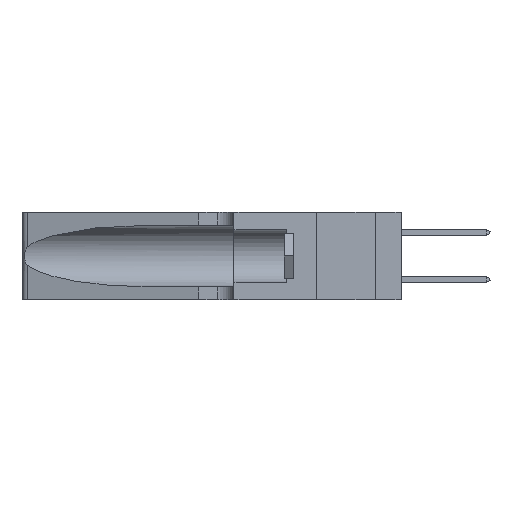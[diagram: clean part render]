
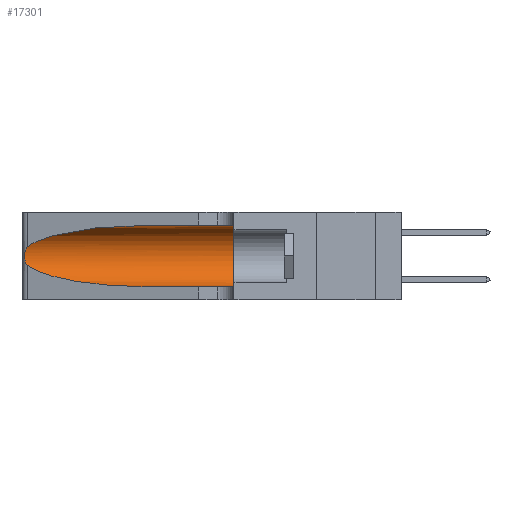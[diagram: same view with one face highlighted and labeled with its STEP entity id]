
A CAD part, left-side view. The second image highlights one B-rep face of the part: STEP entity #17301.
In plain terms, the highlighted cylindrical face has radius 3.308 mm (diameter 6.617 mm), a partial arc.
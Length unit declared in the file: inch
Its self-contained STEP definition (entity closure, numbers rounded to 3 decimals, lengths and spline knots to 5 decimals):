
#1300 = LINE ( 'NONE', #16439, #38220 ) ;
#2015 = VERTEX_POINT ( 'NONE', #31991 ) ;
#2407 = DIRECTION ( 'NONE',  ( 0., -1., 0. ) ) ;
#2857 = CARTESIAN_POINT ( 'NONE',  ( 0.26017, 1.23833, 0.17102 ) ) ;
#2988 = VECTOR ( 'NONE', #34786, 39.37008 ) ;
#3005 = CARTESIAN_POINT ( 'NONE',  ( 0.25555, 1.22994, 0.2215 ) ) ;
#3020 = ORIENTED_EDGE ( 'NONE', *, *, #15804, .T. ) ;
#4211 = ORIENTED_EDGE ( 'NONE', *, *, #12583, .T. ) ;
#4261 = VERTEX_POINT ( 'NONE', #44285 ) ;
#5601 = CARTESIAN_POINT ( 'NONE',  ( 0.1305, 1.61858, 0.185 ) ) ;
#5669 = ORIENTED_EDGE ( 'NONE', *, *, #14923, .F. ) ;
#6293 = LINE ( 'NONE', #26968, #2988 ) ;
#6396 = CARTESIAN_POINT ( 'NONE',  ( 0.25639, 1.23186, 0.15144 ) ) ;
#6546 = CARTESIAN_POINT ( 'NONE',  ( 0.25854, 1.2359, 0.20912 ) ) ;
#6936 = FACE_OUTER_BOUND ( 'NONE', #11433, .T. ) ;
#9191 = CARTESIAN_POINT ( 'NONE',  ( 0.25487, 1.22718, 0.22369 ) ) ;
#9801 = CARTESIAN_POINT ( 'NONE',  ( 0.26075, 1.23896, 0.19203 ) ) ;
#9802 = CARTESIAN_POINT ( 'NONE',  ( 0.2373, 1.15595, 0.08982 ) ) ;
#9939 = CARTESIAN_POINT ( 'NONE',  ( 0.26075, 1.23896, 0.178 ) ) ;
#10091 = CARTESIAN_POINT ( 'NONE',  ( 0.26018, 1.23835, 0.19895 ) ) ;
#11433 = EDGE_LOOP ( 'NONE', ( #41854, #37205, #3020, #4211, #5669, #37146 ) ) ;
#12000 = CARTESIAN_POINT ( 'NONE',  ( 0.18966, 0.96281, 0.31525 ) ) ;
#12583 = EDGE_CURVE ( 'NONE', #2015, #4261, #6293, .T. ) ;
#14911 = CARTESIAN_POINT ( 'NONE',  ( 0.1305, 0.35, 0.185 ) ) ;
#14923 = EDGE_CURVE ( 'NONE', #27778, #4261, #41966, .T. ) ;
#15804 = EDGE_CURVE ( 'NONE', #37887, #2015, #36014, .T. ) ;
#16439 = CARTESIAN_POINT ( 'NONE',  ( 0.1305, 1.61858, 0.31525 ) ) ;
#16723 = CARTESIAN_POINT ( 'NONE',  ( 0.25487, 1.22718, 0.14631 ) ) ;
#17042 = CARTESIAN_POINT ( 'NONE',  ( 0.25787, 1.23484, 0.2124 ) ) ;
#17301 = ADVANCED_FACE ( 'NONE', ( #6936 ), #27846, .F. ) ;
#19081 = CARTESIAN_POINT ( 'NONE',  ( 0.2373, 1.15595, 0.28018 ) ) ;
#20549 = CARTESIAN_POINT ( 'NONE',  ( 0.25555, 1.22993, 0.14849 ) ) ;
#23751 = CARTESIAN_POINT ( 'NONE',  ( 0.18966, 0.96281, 0.05475 ) ) ;
#24031 = EDGE_CURVE ( 'NONE', #30399, #37887, #25258, .T. ) ;
#24132 = CARTESIAN_POINT ( 'NONE',  ( 0.1305, 0.35, 0.31525 ) ) ;
#25122 = AXIS2_PLACEMENT_3D ( 'NONE', #5601, #30185, #33725 ) ;
#25258 = B_SPLINE_CURVE_WITH_KNOTS ( 'NONE', 3,
 ( #31151, #3005, #27597, #17042, #6546, #10091, #9801, #9939, #2857, #34396, #27445, #6396, #20549, #27290 ),
 .UNSPECIFIED., .F., .F.,
 ( 4, 2, 2, 2, 2, 2, 4 ),
 ( 0., 0.00027, 0.00053, 0.00107, 0.0016, 0.00187, 0.00214 ),
 .UNSPECIFIED. ) ;
#26968 = CARTESIAN_POINT ( 'NONE',  ( 0.1305, 1.61858, 0.05475 ) ) ;
#27290 = CARTESIAN_POINT ( 'NONE',  ( 0.25487, 1.22718, 0.14631 ) ) ;
#27445 = CARTESIAN_POINT ( 'NONE',  ( 0.25789, 1.23486, 0.15765 ) ) ;
#27597 = CARTESIAN_POINT ( 'NONE',  ( 0.25639, 1.23184, 0.21858 ) ) ;
#27778 = VERTEX_POINT ( 'NONE', #24132 ) ;
#27846 = CYLINDRICAL_SURFACE ( 'NONE', #25122, 0.13025 ) ;
#30185 = DIRECTION ( 'NONE',  ( 0., -1., 0. ) ) ;
#30399 = VERTEX_POINT ( 'NONE', #34757 ) ;
#31151 = CARTESIAN_POINT ( 'NONE',  ( 0.25487, 1.22718, 0.22369 ) ) ;
#31991 = CARTESIAN_POINT ( 'NONE',  ( 0.1305, 0.72297, 0.05475 ) ) ;
#32100 = DIRECTION ( 'NONE',  ( 0., 0., 1. ) ) ;
#33725 = DIRECTION ( 'NONE',  ( 0., 0., -1. ) ) ;
#33850 = CARTESIAN_POINT ( 'NONE',  ( 0.1305, 0.72297, 0.31525 ) ) ;
#34393 = VERTEX_POINT ( 'NONE', #33850 ) ;
#34396 = CARTESIAN_POINT ( 'NONE',  ( 0.25856, 1.23593, 0.16098 ) ) ;
#34544 = CARTESIAN_POINT ( 'NONE',  ( 0.1305, 0.72297, 0.05475 ) ) ;
#34757 = CARTESIAN_POINT ( 'NONE',  ( 0.25487, 1.22718, 0.22369 ) ) ;
#34786 = DIRECTION ( 'NONE',  ( 0., -1., 0. ) ) ;
#36014 =( BOUNDED_CURVE ( )  B_SPLINE_CURVE ( 3, ( #41251, #9802, #23751, #34544 ),
 .UNSPECIFIED., .F., .F. ) 
 B_SPLINE_CURVE_WITH_KNOTS ( ( 4, 4 ),
 ( 3.44316, 4.71239 ),
 .UNSPECIFIED. ) 
 CURVE ( )  GEOMETRIC_REPRESENTATION_ITEM ( )  RATIONAL_B_SPLINE_CURVE ( ( 1., 0.87, 0.87, 1. ) ) 
 REPRESENTATION_ITEM ( '' )  );
#37146 = ORIENTED_EDGE ( 'NONE', *, *, #45441, .F. ) ;
#37205 = ORIENTED_EDGE ( 'NONE', *, *, #24031, .T. ) ;
#37887 = VERTEX_POINT ( 'NONE', #16723 ) ;
#38220 = VECTOR ( 'NONE', #2407, 39.37008 ) ;
#39574 = DIRECTION ( 'NONE',  ( 0., 1., 0. ) ) ;
#40181 = CARTESIAN_POINT ( 'NONE',  ( 0.1305, 0.72297, 0.31525 ) ) ;
#41251 = CARTESIAN_POINT ( 'NONE',  ( 0.25487, 1.22718, 0.14631 ) ) ;
#41854 = ORIENTED_EDGE ( 'NONE', *, *, #43246, .T. ) ;
#41966 = CIRCLE ( 'NONE', #44738, 0.13025 ) ;
#42274 =( BOUNDED_CURVE ( )  B_SPLINE_CURVE ( 3, ( #40181, #12000, #19081, #9191 ),
 .UNSPECIFIED., .F., .F. ) 
 B_SPLINE_CURVE_WITH_KNOTS ( ( 4, 4 ),
 ( 1.5708, 2.84003 ),
 .UNSPECIFIED. ) 
 CURVE ( )  GEOMETRIC_REPRESENTATION_ITEM ( )  RATIONAL_B_SPLINE_CURVE ( ( 1., 0.87, 0.87, 1. ) ) 
 REPRESENTATION_ITEM ( '' )  );
#43246 = EDGE_CURVE ( 'NONE', #34393, #30399, #42274, .T. ) ;
#44285 = CARTESIAN_POINT ( 'NONE',  ( 0.1305, 0.35, 0.05475 ) ) ;
#44738 = AXIS2_PLACEMENT_3D ( 'NONE', #14911, #39574, #32100 ) ;
#45441 = EDGE_CURVE ( 'NONE', #34393, #27778, #1300, .T. ) ;
